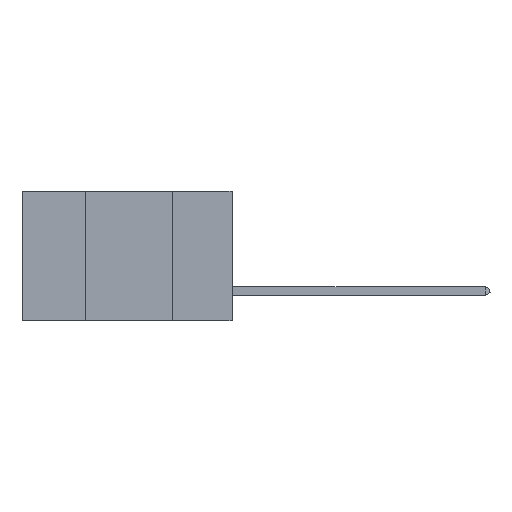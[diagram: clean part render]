
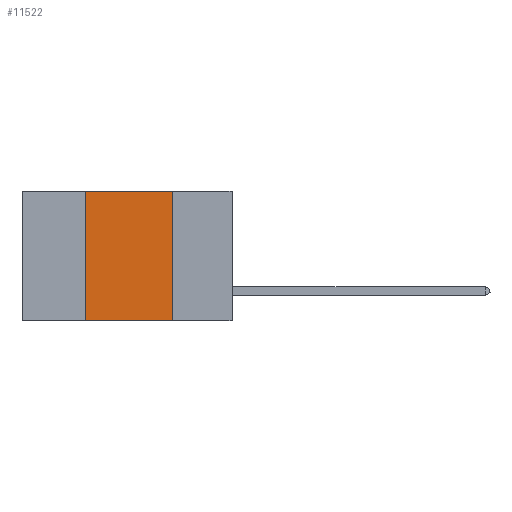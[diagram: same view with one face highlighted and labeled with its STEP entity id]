
A CAD part, left-side view. The second image highlights one B-rep face of the part: STEP entity #11522.
In plain terms, the highlighted planar face has unit normal (-1, 0, 0).
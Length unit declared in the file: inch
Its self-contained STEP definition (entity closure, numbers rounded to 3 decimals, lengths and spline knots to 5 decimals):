
#729 = EDGE_CURVE ( 'NONE', #4639, #824, #7104, .T. ) ;
#824 = VERTEX_POINT ( 'NONE', #11995 ) ;
#1057 = VERTEX_POINT ( 'NONE', #2632 ) ;
#1462 = ORIENTED_EDGE ( 'NONE', *, *, #8242, .T. ) ;
#1655 = LINE ( 'NONE', #2558, #11140 ) ;
#1659 = CARTESIAN_POINT ( 'NONE',  ( 0., 0.17, 0. ) ) ;
#1872 = ORIENTED_EDGE ( 'NONE', *, *, #9331, .F. ) ;
#2229 = CARTESIAN_POINT ( 'NONE',  ( 0., 0.42, 0. ) ) ;
#2558 = CARTESIAN_POINT ( 'NONE',  ( 0., 0.6, 0. ) ) ;
#2632 = CARTESIAN_POINT ( 'NONE',  ( 0., 0.42, -0.37 ) ) ;
#2810 = DIRECTION ( 'NONE',  ( 0., 0., -1. ) ) ;
#3010 = VECTOR ( 'NONE', #2810, 39.37008 ) ;
#3045 = DIRECTION ( 'NONE',  ( 0., -1., 0. ) ) ;
#3764 = VECTOR ( 'NONE', #4336, 39.37008 ) ;
#4336 = DIRECTION ( 'NONE',  ( 0., 0., 1. ) ) ;
#4495 = AXIS2_PLACEMENT_3D ( 'NONE', #11416, #10443, #13451 ) ;
#4639 = VERTEX_POINT ( 'NONE', #5633 ) ;
#5633 = CARTESIAN_POINT ( 'NONE',  ( 0., 0.17, 0. ) ) ;
#6170 = ORIENTED_EDGE ( 'NONE', *, *, #729, .F. ) ;
#6552 = DIRECTION ( 'NONE',  ( 0., -1., 0. ) ) ;
#7104 = LINE ( 'NONE', #1659, #3010 ) ;
#7199 = LINE ( 'NONE', #2229, #3764 ) ;
#8052 = PLANE ( 'NONE',  #4495 ) ;
#8241 = EDGE_LOOP ( 'NONE', ( #6170, #11012, #1872, #1462 ) ) ;
#8242 = EDGE_CURVE ( 'NONE', #1057, #824, #10036, .T. ) ;
#8770 = VERTEX_POINT ( 'NONE', #13463 ) ;
#9317 = CARTESIAN_POINT ( 'NONE',  ( 0., 0.6, -0.37 ) ) ;
#9331 = EDGE_CURVE ( 'NONE', #1057, #8770, #7199, .T. ) ;
#10036 = LINE ( 'NONE', #9317, #13478 ) ;
#10232 = FACE_OUTER_BOUND ( 'NONE', #8241, .T. ) ;
#10443 = DIRECTION ( 'NONE',  ( 1., 0., 0. ) ) ;
#11012 = ORIENTED_EDGE ( 'NONE', *, *, #12929, .F. ) ;
#11140 = VECTOR ( 'NONE', #6552, 39.37008 ) ;
#11416 = CARTESIAN_POINT ( 'NONE',  ( 0., 0.6, 0. ) ) ;
#11522 = ADVANCED_FACE ( 'NONE', ( #10232 ), #8052, .F. ) ;
#11995 = CARTESIAN_POINT ( 'NONE',  ( 0., 0.17, -0.37 ) ) ;
#12929 = EDGE_CURVE ( 'NONE', #8770, #4639, #1655, .T. ) ;
#13451 = DIRECTION ( 'NONE',  ( 0., 0., -1. ) ) ;
#13463 = CARTESIAN_POINT ( 'NONE',  ( 0., 0.42, 0. ) ) ;
#13478 = VECTOR ( 'NONE', #3045, 39.37008 ) ;
